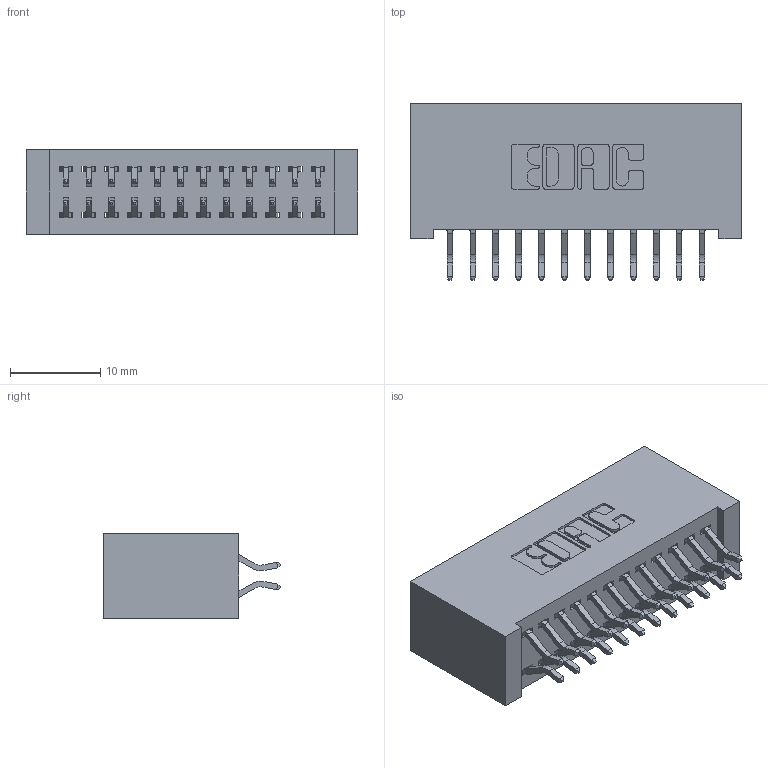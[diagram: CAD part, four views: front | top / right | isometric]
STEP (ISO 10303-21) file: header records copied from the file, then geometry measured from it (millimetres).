
FILE_DESCRIPTION (( 'STEP AP203' ), '1' );
FILE_NAME ('392-024-556-201.STEP', '2019-10-07T07:41:05', ( '' ), ( '' ), 'SwSTEP 2.0', 'SolidWorks 2016', '' );
FILE_SCHEMA (( 'CONFIG_CONTROL_DESIGN' ));
Length unit declared in the file: inch
Products named in the file (3): 342 Part_Lugless; 345-292-001_556 Tail; 392-024-556-201
Assembly tree (25 placements, depth 2):
  392-024-556-201
    342 Part_Lugless
    345-292-001_556 Tail  x24
Bounding box: 36.73 x 19.58 x 9.4 mm (x, y, z)
Volume: 3596.9 mm3; surface area: 5538.7 mm2
Topology: 25 solids, 25 shells, 1494 faces, 4427 edges, 2918 vertices
Faces by surface type: plane 1022, cylinder 472
Entity records: 11411 total; most frequent: CARTESIAN_POINT 1938, ORIENTED_EDGE 1862, DIRECTION 1691, EDGE_CURVE 931, VECTOR 803, LINE 803, VERTEX_POINT 618, AXIS2_PLACEMENT_3D 444
